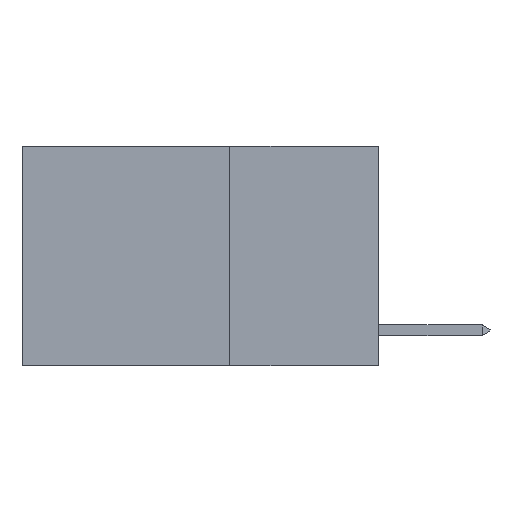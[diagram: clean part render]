
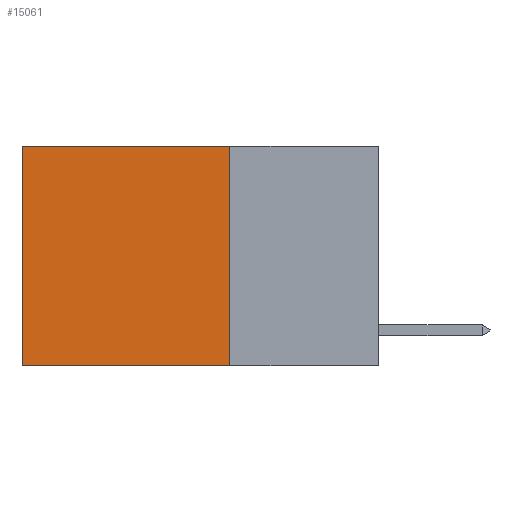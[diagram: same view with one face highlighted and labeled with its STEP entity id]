
A CAD part, left-side view. The second image highlights one B-rep face of the part: STEP entity #15061.
In plain terms, the highlighted planar face has unit normal (-1, 0, 0).
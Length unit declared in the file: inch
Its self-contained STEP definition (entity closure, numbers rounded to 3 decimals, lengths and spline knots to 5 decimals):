
#822 = ORIENTED_EDGE ( 'NONE', *, *, #3057, .T. ) ;
#2405 = VERTEX_POINT ( 'NONE', #6295 ) ;
#3015 = VECTOR ( 'NONE', #7855, 39.37008 ) ;
#3057 = EDGE_CURVE ( 'NONE', #14216, #11108, #13227, .T. ) ;
#3459 = LINE ( 'NONE', #3551, #10815 ) ;
#3551 = CARTESIAN_POINT ( 'NONE',  ( 0.2625, 0.6, 0. ) ) ;
#3607 = CARTESIAN_POINT ( 'NONE',  ( 0.2625, 0.25, -0.37 ) ) ;
#5056 = VECTOR ( 'NONE', #13586, 39.37008 ) ;
#6295 = CARTESIAN_POINT ( 'NONE',  ( 0.2625, 0.6, -0.37 ) ) ;
#6588 = CARTESIAN_POINT ( 'NONE',  ( 0.2625, 0.6, 0. ) ) ;
#6807 = ORIENTED_EDGE ( 'NONE', *, *, #8895, .F. ) ;
#7403 = CARTESIAN_POINT ( 'NONE',  ( 0.2625, 0.25, -0.37 ) ) ;
#7855 = DIRECTION ( 'NONE',  ( 0., 1., 0. ) ) ;
#7955 = CARTESIAN_POINT ( 'NONE',  ( 0.2625, 0.25, 0. ) ) ;
#8139 = DIRECTION ( 'NONE',  ( 0., 0., -1. ) ) ;
#8324 = EDGE_CURVE ( 'NONE', #17197, #2405, #15675, .T. ) ;
#8895 = EDGE_CURVE ( 'NONE', #14216, #17197, #12015, .T. ) ;
#8927 = DIRECTION ( 'NONE',  ( 0., 0., -1. ) ) ;
#9314 = FACE_OUTER_BOUND ( 'NONE', #13093, .T. ) ;
#10622 = PLANE ( 'NONE',  #14467 ) ;
#10815 = VECTOR ( 'NONE', #8927, 39.37008 ) ;
#11108 = VERTEX_POINT ( 'NONE', #6588 ) ;
#11913 = CARTESIAN_POINT ( 'NONE',  ( 0.2625, 0.25, 0. ) ) ;
#12015 = LINE ( 'NONE', #7955, #5056 ) ;
#12419 = ORIENTED_EDGE ( 'NONE', *, *, #15709, .T. ) ;
#12996 = DIRECTION ( 'NONE',  ( 0., 1., 0. ) ) ;
#13093 = EDGE_LOOP ( 'NONE', ( #12419, #15657, #6807, #822 ) ) ;
#13227 = LINE ( 'NONE', #11913, #3015 ) ;
#13586 = DIRECTION ( 'NONE',  ( 0., 0., -1. ) ) ;
#14216 = VERTEX_POINT ( 'NONE', #17126 ) ;
#14467 = AXIS2_PLACEMENT_3D ( 'NONE', #14921, #17232, #8139 ) ;
#14921 = CARTESIAN_POINT ( 'NONE',  ( 0.2625, 0.25, 0. ) ) ;
#15061 = ADVANCED_FACE ( 'NONE', ( #9314 ), #10622, .F. ) ;
#15657 = ORIENTED_EDGE ( 'NONE', *, *, #8324, .F. ) ;
#15675 = LINE ( 'NONE', #3607, #17154 ) ;
#15709 = EDGE_CURVE ( 'NONE', #11108, #2405, #3459, .T. ) ;
#17126 = CARTESIAN_POINT ( 'NONE',  ( 0.2625, 0.25, 0. ) ) ;
#17154 = VECTOR ( 'NONE', #12996, 39.37008 ) ;
#17197 = VERTEX_POINT ( 'NONE', #7403 ) ;
#17232 = DIRECTION ( 'NONE',  ( 1., 0., 0. ) ) ;
